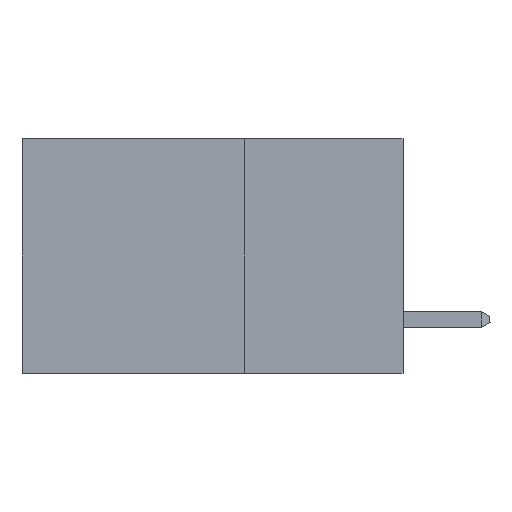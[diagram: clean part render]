
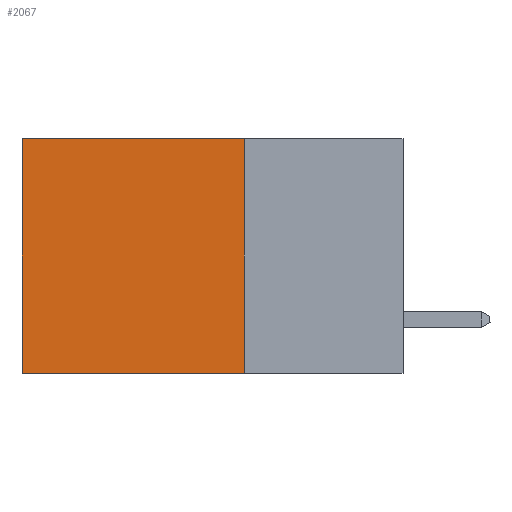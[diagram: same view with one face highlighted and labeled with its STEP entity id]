
A CAD part, left-side view. The second image highlights one B-rep face of the part: STEP entity #2067.
In plain terms, the highlighted planar face has unit normal (-1, 0, 0).
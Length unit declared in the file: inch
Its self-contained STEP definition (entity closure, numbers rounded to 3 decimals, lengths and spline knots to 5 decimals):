
#130 = CARTESIAN_POINT ( 'NONE',  ( 0.2875, 0.25, 0. ) ) ;
#602 = CARTESIAN_POINT ( 'NONE',  ( 0.2875, 0.25, -0.37 ) ) ;
#991 = VERTEX_POINT ( 'NONE', #2702 ) ;
#1631 = EDGE_CURVE ( 'NONE', #3710, #3467, #2881, .T. ) ;
#2067 = ADVANCED_FACE ( 'NONE', ( #14196 ), #20011, .F. ) ;
#2142 = ORIENTED_EDGE ( 'NONE', *, *, #18660, .T. ) ;
#2280 = CARTESIAN_POINT ( 'NONE',  ( 0.2875, 0.25, -0.37 ) ) ;
#2702 = CARTESIAN_POINT ( 'NONE',  ( 0.2875, 0.6, 0. ) ) ;
#2706 = CARTESIAN_POINT ( 'NONE',  ( 0.2875, 0.25, 0. ) ) ;
#2881 = LINE ( 'NONE', #2706, #9655 ) ;
#3467 = VERTEX_POINT ( 'NONE', #602 ) ;
#3710 = VERTEX_POINT ( 'NONE', #5594 ) ;
#5594 = CARTESIAN_POINT ( 'NONE',  ( 0.2875, 0.25, 0. ) ) ;
#5701 = DIRECTION ( 'NONE',  ( 0., 1., 0. ) ) ;
#6113 = CARTESIAN_POINT ( 'NONE',  ( 0.2875, 0.25, 0. ) ) ;
#6470 = VECTOR ( 'NONE', #5701, 39.37008 ) ;
#7457 = CARTESIAN_POINT ( 'NONE',  ( 0.2875, 0.6, 0. ) ) ;
#8033 = EDGE_LOOP ( 'NONE', ( #11045, #18588, #20411, #2142 ) ) ;
#9655 = VECTOR ( 'NONE', #16483, 39.37008 ) ;
#10827 = CARTESIAN_POINT ( 'NONE',  ( 0.2875, 0.6, -0.37 ) ) ;
#11045 = ORIENTED_EDGE ( 'NONE', *, *, #21810, .T. ) ;
#11586 = DIRECTION ( 'NONE',  ( 1., 0., 0. ) ) ;
#12962 = DIRECTION ( 'NONE',  ( 0., 0., -1. ) ) ;
#14196 = FACE_OUTER_BOUND ( 'NONE', #8033, .T. ) ;
#14474 = EDGE_CURVE ( 'NONE', #3467, #17479, #21248, .T. ) ;
#14947 = AXIS2_PLACEMENT_3D ( 'NONE', #6113, #11586, #12962 ) ;
#15629 = LINE ( 'NONE', #130, #6470 ) ;
#16483 = DIRECTION ( 'NONE',  ( 0., 0., -1. ) ) ;
#16643 = VECTOR ( 'NONE', #19391, 39.37008 ) ;
#17479 = VERTEX_POINT ( 'NONE', #10827 ) ;
#17893 = DIRECTION ( 'NONE',  ( 0., 0., -1. ) ) ;
#17907 = VECTOR ( 'NONE', #17893, 39.37008 ) ;
#18588 = ORIENTED_EDGE ( 'NONE', *, *, #14474, .F. ) ;
#18656 = LINE ( 'NONE', #7457, #17907 ) ;
#18660 = EDGE_CURVE ( 'NONE', #3710, #991, #15629, .T. ) ;
#19391 = DIRECTION ( 'NONE',  ( 0., 1., 0. ) ) ;
#20011 = PLANE ( 'NONE',  #14947 ) ;
#20411 = ORIENTED_EDGE ( 'NONE', *, *, #1631, .F. ) ;
#21248 = LINE ( 'NONE', #2280, #16643 ) ;
#21810 = EDGE_CURVE ( 'NONE', #991, #17479, #18656, .T. ) ;
